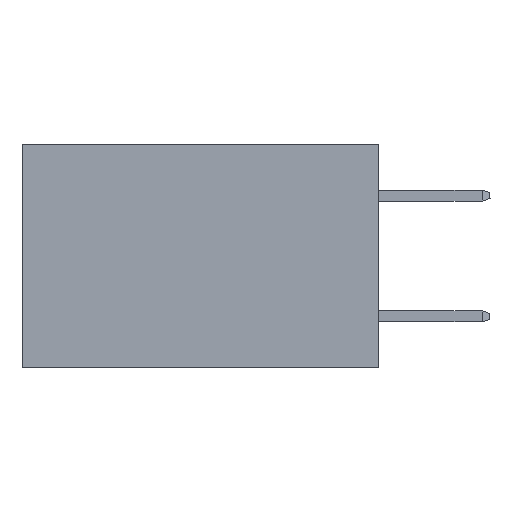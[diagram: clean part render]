
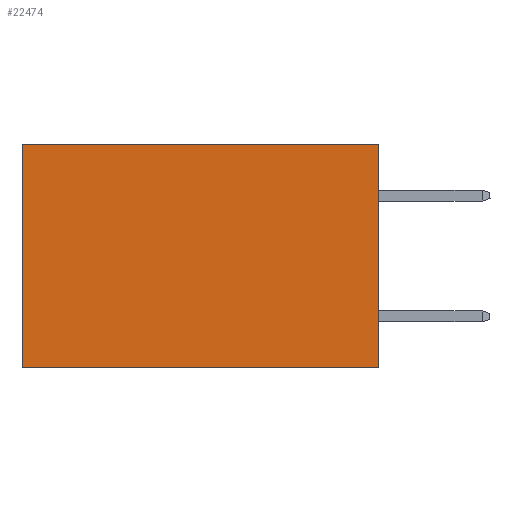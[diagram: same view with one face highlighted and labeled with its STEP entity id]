
A CAD part, left-side view. The second image highlights one B-rep face of the part: STEP entity #22474.
In plain terms, the highlighted planar face has unit normal (-1, 0, 0).
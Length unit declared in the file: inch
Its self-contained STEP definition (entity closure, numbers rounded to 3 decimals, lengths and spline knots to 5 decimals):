
#1383 = EDGE_CURVE ( 'NONE', #13068, #11976, #5784, .T. ) ;
#2816 = FACE_OUTER_BOUND ( 'NONE', #28423, .T. ) ;
#3518 = AXIS2_PLACEMENT_3D ( 'NONE', #19904, #5676, #22271 ) ;
#4858 = DIRECTION ( 'NONE',  ( 0., 1., 0. ) ) ;
#5676 = DIRECTION ( 'NONE',  ( 1., 0., 0. ) ) ;
#5784 = LINE ( 'NONE', #19043, #11403 ) ;
#6305 = CARTESIAN_POINT ( 'NONE',  ( 0.277, 0., -0.37 ) ) ;
#7164 = VECTOR ( 'NONE', #4858, 39.37008 ) ;
#8152 = ORIENTED_EDGE ( 'NONE', *, *, #12719, .F. ) ;
#8842 = CARTESIAN_POINT ( 'NONE',  ( 0.277, 0., -0.37 ) ) ;
#9625 = DIRECTION ( 'NONE',  ( 0., 0., -1. ) ) ;
#11403 = VECTOR ( 'NONE', #9625, 39.37008 ) ;
#11653 = CARTESIAN_POINT ( 'NONE',  ( 0.277, 0., 0. ) ) ;
#11976 = VERTEX_POINT ( 'NONE', #15281 ) ;
#12244 = LINE ( 'NONE', #8842, #24094 ) ;
#12719 = EDGE_CURVE ( 'NONE', #30576, #11976, #25801, .T. ) ;
#12853 = ORIENTED_EDGE ( 'NONE', *, *, #1383, .T. ) ;
#13068 = VERTEX_POINT ( 'NONE', #28716 ) ;
#14147 = ORIENTED_EDGE ( 'NONE', *, *, #15904, .T. ) ;
#15281 = CARTESIAN_POINT ( 'NONE',  ( 0.277, 0.59, -0.37 ) ) ;
#15904 = EDGE_CURVE ( 'NONE', #25676, #13068, #26040, .T. ) ;
#18240 = DIRECTION ( 'NONE',  ( 0., 1., 0. ) ) ;
#19043 = CARTESIAN_POINT ( 'NONE',  ( 0.277, 0.59, -0.37 ) ) ;
#19515 = VECTOR ( 'NONE', #18240, 39.37008 ) ;
#19904 = CARTESIAN_POINT ( 'NONE',  ( 0.277, 0., -0.37 ) ) ;
#22271 = DIRECTION ( 'NONE',  ( 0., 0., -1. ) ) ;
#22474 = ADVANCED_FACE ( 'NONE', ( #2816 ), #26917, .F. ) ;
#24094 = VECTOR ( 'NONE', #25379, 39.37008 ) ;
#25379 = DIRECTION ( 'NONE',  ( 0., 0., -1. ) ) ;
#25676 = VERTEX_POINT ( 'NONE', #11653 ) ;
#25801 = LINE ( 'NONE', #6305, #19515 ) ;
#26040 = LINE ( 'NONE', #26244, #7164 ) ;
#26244 = CARTESIAN_POINT ( 'NONE',  ( 0.277, 0., 0. ) ) ;
#26917 = PLANE ( 'NONE',  #3518 ) ;
#28178 = ORIENTED_EDGE ( 'NONE', *, *, #28439, .F. ) ;
#28423 = EDGE_LOOP ( 'NONE', ( #12853, #8152, #28178, #14147 ) ) ;
#28439 = EDGE_CURVE ( 'NONE', #25676, #30576, #12244, .T. ) ;
#28716 = CARTESIAN_POINT ( 'NONE',  ( 0.277, 0.59, 0. ) ) ;
#29548 = CARTESIAN_POINT ( 'NONE',  ( 0.277, 0., -0.37 ) ) ;
#30576 = VERTEX_POINT ( 'NONE', #29548 ) ;
